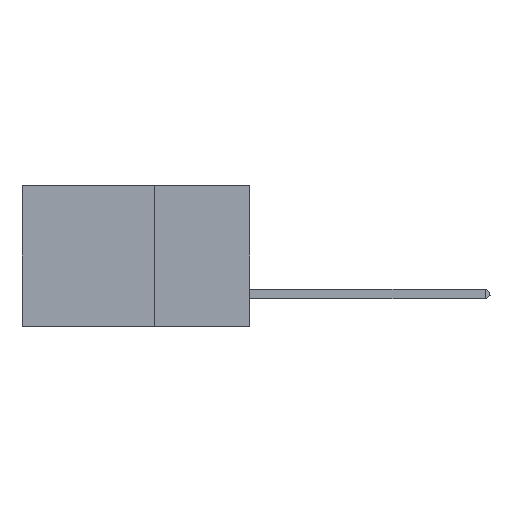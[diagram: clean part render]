
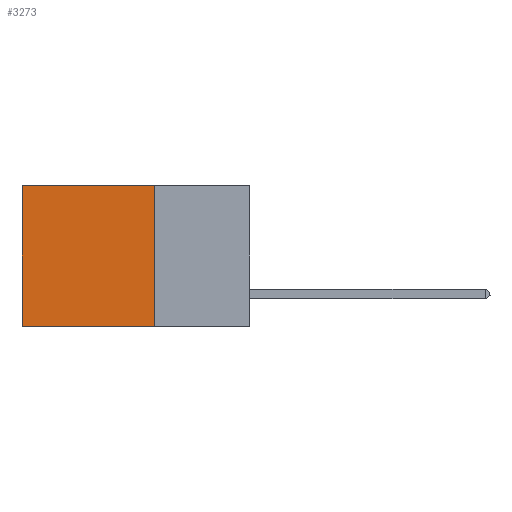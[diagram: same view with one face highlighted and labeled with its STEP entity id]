
A CAD part, left-side view. The second image highlights one B-rep face of the part: STEP entity #3273.
In plain terms, the highlighted planar face has unit normal (-1, 0, 0).
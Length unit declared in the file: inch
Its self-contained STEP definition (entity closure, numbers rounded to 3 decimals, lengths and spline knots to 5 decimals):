
#2170 = FACE_OUTER_BOUND ( 'NONE', #46564, .T. ) ;
#3273 = ADVANCED_FACE ( 'NONE', ( #2170 ), #43758, .F. ) ;
#3653 = EDGE_CURVE ( 'NONE', #32751, #45231, #6858, .T. ) ;
#3940 = VERTEX_POINT ( 'NONE', #19635 ) ;
#4941 = VECTOR ( 'NONE', #39690, 39.37008 ) ;
#5717 = CARTESIAN_POINT ( 'NONE',  ( 0.2875, 0.25, 0. ) ) ;
#6858 = LINE ( 'NONE', #42991, #10427 ) ;
#6925 = DIRECTION ( 'NONE',  ( 0., 0., -1. ) ) ;
#8829 = VECTOR ( 'NONE', #26123, 39.37008 ) ;
#10427 = VECTOR ( 'NONE', #27799, 39.37008 ) ;
#11360 = ORIENTED_EDGE ( 'NONE', *, *, #23563, .T. ) ;
#15065 = CARTESIAN_POINT ( 'NONE',  ( 0.2875, 0.6, 0. ) ) ;
#15322 = LINE ( 'NONE', #15065, #8829 ) ;
#16630 = CARTESIAN_POINT ( 'NONE',  ( 0.2875, 0.6, -0.37 ) ) ;
#16978 = EDGE_CURVE ( 'NONE', #37886, #45231, #15322, .T. ) ;
#19635 = CARTESIAN_POINT ( 'NONE',  ( 0.2875, 0.25, 0. ) ) ;
#23563 = EDGE_CURVE ( 'NONE', #3940, #37886, #41615, .T. ) ;
#26123 = DIRECTION ( 'NONE',  ( 0., 0., -1. ) ) ;
#27249 = ORIENTED_EDGE ( 'NONE', *, *, #16978, .T. ) ;
#27403 = AXIS2_PLACEMENT_3D ( 'NONE', #30869, #46533, #6925 ) ;
#27799 = DIRECTION ( 'NONE',  ( 0., 1., 0. ) ) ;
#28590 = CARTESIAN_POINT ( 'NONE',  ( 0.2875, 0.6, 0. ) ) ;
#28739 = EDGE_CURVE ( 'NONE', #3940, #32751, #45938, .T. ) ;
#30205 = ORIENTED_EDGE ( 'NONE', *, *, #3653, .F. ) ;
#30869 = CARTESIAN_POINT ( 'NONE',  ( 0.2875, 0.25, 0. ) ) ;
#32673 = ORIENTED_EDGE ( 'NONE', *, *, #28739, .F. ) ;
#32751 = VERTEX_POINT ( 'NONE', #47376 ) ;
#34983 = DIRECTION ( 'NONE',  ( 0., 0., -1. ) ) ;
#37886 = VERTEX_POINT ( 'NONE', #28590 ) ;
#39690 = DIRECTION ( 'NONE',  ( 0., 1., 0. ) ) ;
#41615 = LINE ( 'NONE', #5717, #4941 ) ;
#42346 = VECTOR ( 'NONE', #34983, 39.37008 ) ;
#42991 = CARTESIAN_POINT ( 'NONE',  ( 0.2875, 0.25, -0.37 ) ) ;
#43758 = PLANE ( 'NONE',  #27403 ) ;
#45231 = VERTEX_POINT ( 'NONE', #16630 ) ;
#45938 = LINE ( 'NONE', #46362, #42346 ) ;
#46362 = CARTESIAN_POINT ( 'NONE',  ( 0.2875, 0.25, 0. ) ) ;
#46533 = DIRECTION ( 'NONE',  ( 1., 0., 0. ) ) ;
#46564 = EDGE_LOOP ( 'NONE', ( #27249, #30205, #32673, #11360 ) ) ;
#47376 = CARTESIAN_POINT ( 'NONE',  ( 0.2875, 0.25, -0.37 ) ) ;
